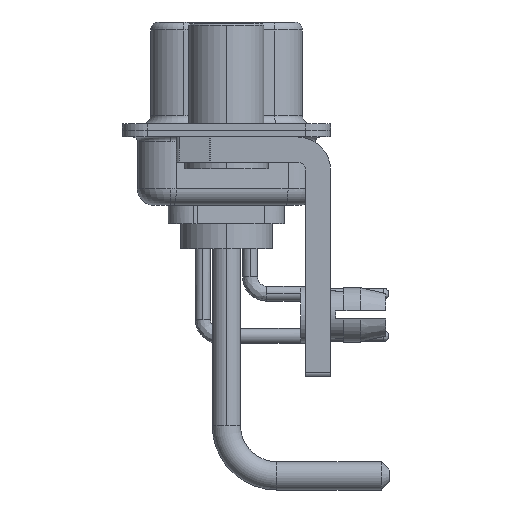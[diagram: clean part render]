
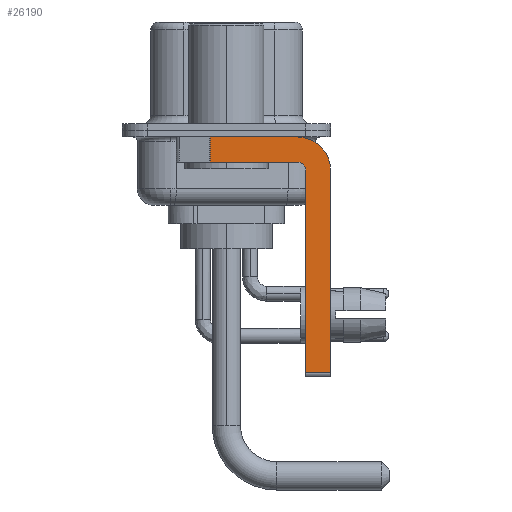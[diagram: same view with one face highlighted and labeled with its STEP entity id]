
A CAD part, left-side view. The second image highlights one B-rep face of the part: STEP entity #26190.
In plain terms, the highlighted planar face has unit normal (-1, 0, 0).
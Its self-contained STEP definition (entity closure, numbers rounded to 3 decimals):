
#146 = EDGE_CURVE ( 'NONE', #13382, #25635, #12149, .T. ) ;
#427 = ORIENTED_EDGE ( 'NONE', *, *, #22669, .F. ) ;
#644 = DIRECTION ( 'NONE',  ( 1., 0., 0. ) ) ;
#896 = LINE ( 'NONE', #3230, #2346 ) ;
#1908 = CARTESIAN_POINT ( 'NONE',  ( -2.9, -6.25, -14.55 ) ) ;
#2325 = LINE ( 'NONE', #13564, #22266 ) ;
#2346 = VECTOR ( 'NONE', #12134, 1000. ) ;
#2365 = CARTESIAN_POINT ( 'NONE',  ( -2.9, -4.25, -1.9 ) ) ;
#3230 = CARTESIAN_POINT ( 'NONE',  ( -2.9, -4.75, -14.8 ) ) ;
#3334 = AXIS2_PLACEMENT_3D ( 'NONE', #21059, #22818, #5131 ) ;
#4860 = VERTEX_POINT ( 'NONE', #22784 ) ;
#5131 = DIRECTION ( 'NONE',  ( 0., 0., -1. ) ) ;
#6613 = LINE ( 'NONE', #22388, #19600 ) ;
#7096 = CARTESIAN_POINT ( 'NONE',  ( -2.9, -4.25, -2.4 ) ) ;
#8486 = ORIENTED_EDGE ( 'NONE', *, *, #12435, .F. ) ;
#8765 = DIRECTION ( 'NONE',  ( 0., -1., 0. ) ) ;
#8879 = DIRECTION ( 'NONE',  ( 0., 0., -1. ) ) ;
#9019 = CIRCLE ( 'NONE', #19306, 0.5 ) ;
#9045 = CARTESIAN_POINT ( 'NONE',  ( -2.9, -4.25, -14.55 ) ) ;
#9373 = CIRCLE ( 'NONE', #3334, 2. ) ;
#9400 = CARTESIAN_POINT ( 'NONE',  ( -2.9, -4.25, -2.4 ) ) ;
#9933 = VERTEX_POINT ( 'NONE', #15446 ) ;
#10627 = EDGE_LOOP ( 'NONE', ( #20586, #17407, #27921, #8486, #12312, #23064, #21805, #427 ) ) ;
#10840 = DIRECTION ( 'NONE',  ( 0., -1., 0. ) ) ;
#12134 = DIRECTION ( 'NONE',  ( 0., 0., 1. ) ) ;
#12149 = LINE ( 'NONE', #12740, #15149 ) ;
#12304 = CARTESIAN_POINT ( 'NONE',  ( -2.9, -6.25, -2.4 ) ) ;
#12312 = ORIENTED_EDGE ( 'NONE', *, *, #21131, .F. ) ;
#12435 = EDGE_CURVE ( 'NONE', #4860, #22011, #9019, .T. ) ;
#12740 = CARTESIAN_POINT ( 'NONE',  ( -2.9, -6.25, -2.4 ) ) ;
#13382 = VERTEX_POINT ( 'NONE', #12304 ) ;
#13564 = CARTESIAN_POINT ( 'NONE',  ( -2.9, 0.978, -1.9 ) ) ;
#13576 = EDGE_CURVE ( 'NONE', #22011, #18762, #24711, .T. ) ;
#13711 = VECTOR ( 'NONE', #15224, 1000. ) ;
#13961 = DIRECTION ( 'NONE',  ( 0., 0., 1. ) ) ;
#14095 = PLANE ( 'NONE',  #27690 ) ;
#15033 = VERTEX_POINT ( 'NONE', #21105 ) ;
#15149 = VECTOR ( 'NONE', #18883, 1000. ) ;
#15224 = DIRECTION ( 'NONE',  ( 0., 1., 0. ) ) ;
#15446 = CARTESIAN_POINT ( 'NONE',  ( -2.9, -4.25, -0.4 ) ) ;
#15848 = DIRECTION ( 'NONE',  ( 0., 0., -1. ) ) ;
#16950 = EDGE_CURVE ( 'NONE', #15033, #25635, #28637, .T. ) ;
#17407 = ORIENTED_EDGE ( 'NONE', *, *, #17975, .T. ) ;
#17975 = EDGE_CURVE ( 'NONE', #21540, #18762, #2325, .T. ) ;
#18762 = VERTEX_POINT ( 'NONE', #23606 ) ;
#18883 = DIRECTION ( 'NONE',  ( 0., 0., -1. ) ) ;
#19306 = AXIS2_PLACEMENT_3D ( 'NONE', #7096, #24915, #13961 ) ;
#19600 = VECTOR ( 'NONE', #10840, 1000. ) ;
#20586 = ORIENTED_EDGE ( 'NONE', *, *, #20830, .F. ) ;
#20830 = EDGE_CURVE ( 'NONE', #21540, #9933, #6613, .T. ) ;
#21059 = CARTESIAN_POINT ( 'NONE',  ( -2.9, -4.25, -2.4 ) ) ;
#21105 = CARTESIAN_POINT ( 'NONE',  ( -2.9, -4.75, -14.55 ) ) ;
#21131 = EDGE_CURVE ( 'NONE', #15033, #4860, #896, .T. ) ;
#21540 = VERTEX_POINT ( 'NONE', #25716 ) ;
#21702 = CARTESIAN_POINT ( 'NONE',  ( -2.9, -4.25, -1.9 ) ) ;
#21805 = ORIENTED_EDGE ( 'NONE', *, *, #146, .F. ) ;
#22011 = VERTEX_POINT ( 'NONE', #21702 ) ;
#22266 = VECTOR ( 'NONE', #8879, 1000. ) ;
#22388 = CARTESIAN_POINT ( 'NONE',  ( -2.9, 3., -0.4 ) ) ;
#22669 = EDGE_CURVE ( 'NONE', #9933, #13382, #9373, .T. ) ;
#22784 = CARTESIAN_POINT ( 'NONE',  ( -2.9, -4.75, -2.4 ) ) ;
#22818 = DIRECTION ( 'NONE',  ( 1., 0., 0. ) ) ;
#23064 = ORIENTED_EDGE ( 'NONE', *, *, #16950, .T. ) ;
#23178 = VECTOR ( 'NONE', #8765, 1000. ) ;
#23606 = CARTESIAN_POINT ( 'NONE',  ( -2.9, 0.978, -1.9 ) ) ;
#24711 = LINE ( 'NONE', #2365, #13711 ) ;
#24915 = DIRECTION ( 'NONE',  ( -1., 0., 0. ) ) ;
#25635 = VERTEX_POINT ( 'NONE', #1908 ) ;
#25716 = CARTESIAN_POINT ( 'NONE',  ( -2.9, 0.978, -0.4 ) ) ;
#26190 = ADVANCED_FACE ( 'NONE', ( #27377 ), #14095, .F. ) ;
#27377 = FACE_OUTER_BOUND ( 'NONE', #10627, .T. ) ;
#27690 = AXIS2_PLACEMENT_3D ( 'NONE', #9400, #644, #15848 ) ;
#27921 = ORIENTED_EDGE ( 'NONE', *, *, #13576, .F. ) ;
#28637 = LINE ( 'NONE', #9045, #23178 ) ;
